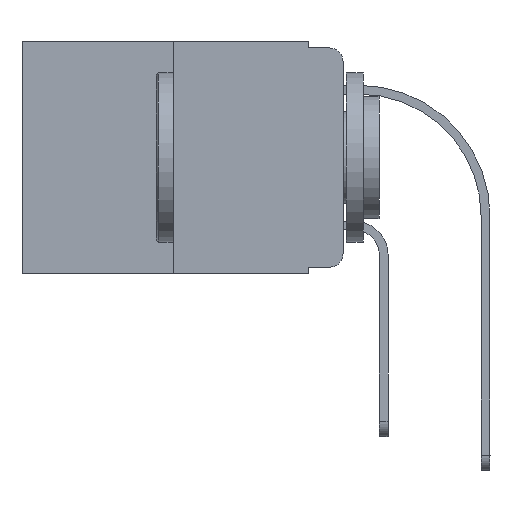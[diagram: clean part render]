
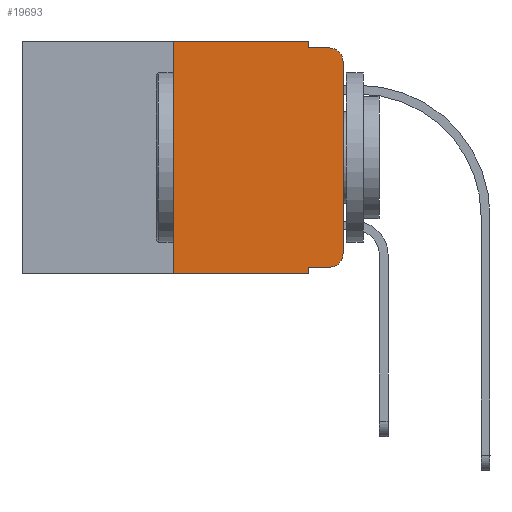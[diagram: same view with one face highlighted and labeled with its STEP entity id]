
A CAD part, left-side view. The second image highlights one B-rep face of the part: STEP entity #19693.
In plain terms, the highlighted planar face has unit normal (-1, 0, 0).
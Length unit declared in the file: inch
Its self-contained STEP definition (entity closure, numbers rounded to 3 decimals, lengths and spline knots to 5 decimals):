
#374 = DIRECTION ( 'NONE',  ( 0., -1., 0. ) ) ;
#891 = EDGE_CURVE ( 'NONE', #12152, #18682, #20447, .T. ) ;
#1131 = EDGE_CURVE ( 'NONE', #17527, #4863, #8953, .T. ) ;
#1152 = CARTESIAN_POINT ( 'NONE',  ( 0., 0.051, -0.333 ) ) ;
#1428 = CARTESIAN_POINT ( 'NONE',  ( 0., 0.473, 0. ) ) ;
#1818 = CARTESIAN_POINT ( 'NONE',  ( 0., 0.051, -0.343 ) ) ;
#2170 = VERTEX_POINT ( 'NONE', #21929 ) ;
#2270 = EDGE_CURVE ( 'NONE', #21619, #11688, #9092, .T. ) ;
#2329 = DIRECTION ( 'NONE',  ( 0., 0., -1. ) ) ;
#2411 = DIRECTION ( 'NONE',  ( 0., 0., -1. ) ) ;
#2923 = LINE ( 'NONE', #18480, #14606 ) ;
#3165 = VECTOR ( 'NONE', #15960, 39.37008 ) ;
#3224 = DIRECTION ( 'NONE',  ( 1., 0., 0. ) ) ;
#3718 = ORIENTED_EDGE ( 'NONE', *, *, #16817, .T. ) ;
#4340 = CARTESIAN_POINT ( 'NONE',  ( 0., 0.051, -0.01 ) ) ;
#4512 = CARTESIAN_POINT ( 'NONE',  ( 0., 0.02, -0.333 ) ) ;
#4751 = ORIENTED_EDGE ( 'NONE', *, *, #21331, .F. ) ;
#4804 = CARTESIAN_POINT ( 'NONE',  ( 0., 0.25, 0. ) ) ;
#4863 = VERTEX_POINT ( 'NONE', #1818 ) ;
#5200 = CARTESIAN_POINT ( 'NONE',  ( 0., 0., -0.03 ) ) ;
#5700 = CARTESIAN_POINT ( 'NONE',  ( 0., 0.02, -0.313 ) ) ;
#6305 = ORIENTED_EDGE ( 'NONE', *, *, #891, .T. ) ;
#6335 = VECTOR ( 'NONE', #374, 39.37008 ) ;
#7046 = PLANE ( 'NONE',  #9140 ) ;
#7282 = CARTESIAN_POINT ( 'NONE',  ( 0., 0.051, 0. ) ) ;
#8619 = EDGE_CURVE ( 'NONE', #2170, #13566, #15044, .T. ) ;
#8698 = CIRCLE ( 'NONE', #11224, 0.02 ) ;
#8953 = LINE ( 'NONE', #15812, #6335 ) ;
#9037 = CARTESIAN_POINT ( 'NONE',  ( 0., 0.25, -0.343 ) ) ;
#9092 = LINE ( 'NONE', #19340, #3165 ) ;
#9140 = AXIS2_PLACEMENT_3D ( 'NONE', #1428, #3224, #13723 ) ;
#9326 = ORIENTED_EDGE ( 'NONE', *, *, #19912, .F. ) ;
#9459 = CARTESIAN_POINT ( 'NONE',  ( 0., 0., -0.313 ) ) ;
#10230 = CARTESIAN_POINT ( 'NONE',  ( 0., 0.051, 0. ) ) ;
#10360 = DIRECTION ( 'NONE',  ( 0., 0., 1. ) ) ;
#10684 = EDGE_LOOP ( 'NONE', ( #14200, #3718, #9326, #10929, #4751, #13757, #10956, #13939, #6305, #19476 ) ) ;
#10865 = AXIS2_PLACEMENT_3D ( 'NONE', #5700, #12608, #2329 ) ;
#10929 = ORIENTED_EDGE ( 'NONE', *, *, #8619, .F. ) ;
#10956 = ORIENTED_EDGE ( 'NONE', *, *, #1131, .T. ) ;
#11224 = AXIS2_PLACEMENT_3D ( 'NONE', #14521, #16417, #11378 ) ;
#11378 = DIRECTION ( 'NONE',  ( 0., 0., -1. ) ) ;
#11688 = VERTEX_POINT ( 'NONE', #5200 ) ;
#11748 = DIRECTION ( 'NONE',  ( 0., -1., 0. ) ) ;
#12152 = VERTEX_POINT ( 'NONE', #1152 ) ;
#12608 = DIRECTION ( 'NONE',  ( -1., 0., 0. ) ) ;
#12743 = VECTOR ( 'NONE', #2411, 39.37008 ) ;
#13000 = CIRCLE ( 'NONE', #10865, 0.02 ) ;
#13027 = DIRECTION ( 'NONE',  ( 0., -1., 0. ) ) ;
#13566 = VERTEX_POINT ( 'NONE', #4340 ) ;
#13723 = DIRECTION ( 'NONE',  ( 0., 0., -1. ) ) ;
#13757 = ORIENTED_EDGE ( 'NONE', *, *, #21943, .F. ) ;
#13939 = ORIENTED_EDGE ( 'NONE', *, *, #19780, .F. ) ;
#14200 = ORIENTED_EDGE ( 'NONE', *, *, #2270, .T. ) ;
#14521 = CARTESIAN_POINT ( 'NONE',  ( 0., 0.02, -0.03 ) ) ;
#14606 = VECTOR ( 'NONE', #11748, 39.37008 ) ;
#14707 = LINE ( 'NONE', #20003, #14912 ) ;
#14912 = VECTOR ( 'NONE', #13027, 39.37008 ) ;
#15044 = LINE ( 'NONE', #10230, #16916 ) ;
#15593 = DIRECTION ( 'NONE',  ( 0., -1., 0. ) ) ;
#15733 = LINE ( 'NONE', #7282, #12743 ) ;
#15812 = CARTESIAN_POINT ( 'NONE',  ( 0., 0.473, -0.343 ) ) ;
#15851 = LINE ( 'NONE', #18901, #20381 ) ;
#15960 = DIRECTION ( 'NONE',  ( 0., 0., 1. ) ) ;
#16417 = DIRECTION ( 'NONE',  ( -1., 0., 0. ) ) ;
#16713 = EDGE_CURVE ( 'NONE', #18682, #21619, #13000, .T. ) ;
#16817 = EDGE_CURVE ( 'NONE', #11688, #19724, #8698, .T. ) ;
#16865 = CARTESIAN_POINT ( 'NONE',  ( 0., 0.02, -0.01 ) ) ;
#16916 = VECTOR ( 'NONE', #21908, 39.37008 ) ;
#16964 = CARTESIAN_POINT ( 'NONE',  ( 0., 0.051, -0.333 ) ) ;
#17527 = VERTEX_POINT ( 'NONE', #9037 ) ;
#18480 = CARTESIAN_POINT ( 'NONE',  ( 0., 0.473, 0. ) ) ;
#18682 = VERTEX_POINT ( 'NONE', #4512 ) ;
#18894 = FACE_OUTER_BOUND ( 'NONE', #10684, .T. ) ;
#18901 = CARTESIAN_POINT ( 'NONE',  ( 0., 0.25, 0. ) ) ;
#19295 = VECTOR ( 'NONE', #15593, 39.37008 ) ;
#19340 = CARTESIAN_POINT ( 'NONE',  ( 0., 0., 0. ) ) ;
#19476 = ORIENTED_EDGE ( 'NONE', *, *, #16713, .T. ) ;
#19693 = ADVANCED_FACE ( 'NONE', ( #18894 ), #7046, .F. ) ;
#19724 = VERTEX_POINT ( 'NONE', #16865 ) ;
#19780 = EDGE_CURVE ( 'NONE', #12152, #4863, #15733, .T. ) ;
#19912 = EDGE_CURVE ( 'NONE', #13566, #19724, #14707, .T. ) ;
#20003 = CARTESIAN_POINT ( 'NONE',  ( 0., 0.051, -0.01 ) ) ;
#20381 = VECTOR ( 'NONE', #10360, 39.37008 ) ;
#20447 = LINE ( 'NONE', #16964, #19295 ) ;
#21331 = EDGE_CURVE ( 'NONE', #21759, #2170, #2923, .T. ) ;
#21619 = VERTEX_POINT ( 'NONE', #9459 ) ;
#21759 = VERTEX_POINT ( 'NONE', #4804 ) ;
#21908 = DIRECTION ( 'NONE',  ( 0., 0., -1. ) ) ;
#21929 = CARTESIAN_POINT ( 'NONE',  ( 0., 0.051, 0. ) ) ;
#21943 = EDGE_CURVE ( 'NONE', #17527, #21759, #15851, .T. ) ;
